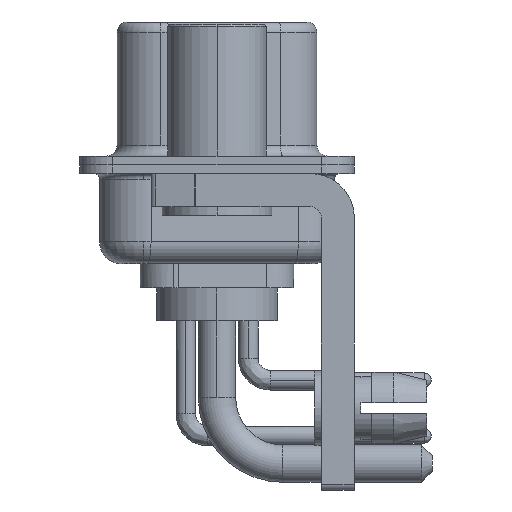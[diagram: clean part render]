
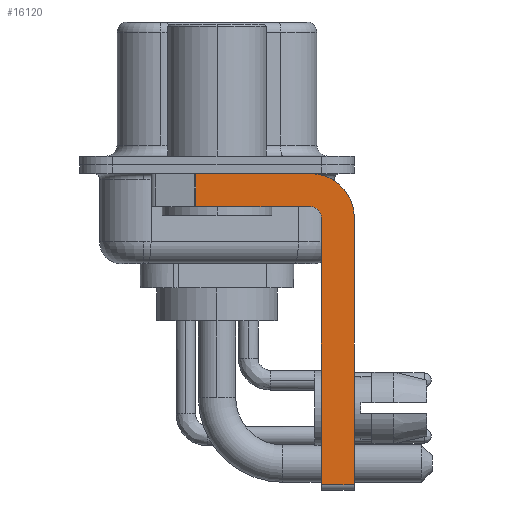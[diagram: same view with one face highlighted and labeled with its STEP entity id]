
A CAD part, left-side view. The second image highlights one B-rep face of the part: STEP entity #16120.
In plain terms, the highlighted planar face has unit normal (-1, 0, 0).
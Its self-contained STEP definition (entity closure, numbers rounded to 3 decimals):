
#442 = PLANE ( 'NONE',  #22238 ) ;
#524 = VECTOR ( 'NONE', #937, 1000. ) ;
#581 = DIRECTION ( 'NONE',  ( 0., 0., -1. ) ) ;
#937 = DIRECTION ( 'NONE',  ( 0., -1., 0. ) ) ;
#1327 = FACE_OUTER_BOUND ( 'NONE', #17227, .T. ) ;
#2246 = EDGE_CURVE ( 'NONE', #13274, #13273, #14665, .T. ) ;
#2663 = CARTESIAN_POINT ( 'NONE',  ( -2.9, -4.75, -2.4 ) ) ;
#3326 = LINE ( 'NONE', #11340, #25984 ) ;
#3501 = EDGE_CURVE ( 'NONE', #24560, #13274, #6571, .T. ) ;
#3505 = CARTESIAN_POINT ( 'NONE',  ( -2.9, -4.75, -14.8 ) ) ;
#3514 = EDGE_CURVE ( 'NONE', #13273, #20298, #10653, .T. ) ;
#4034 = EDGE_CURVE ( 'NONE', #24560, #18613, #13645, .T. ) ;
#4553 = ORIENTED_EDGE ( 'NONE', *, *, #2246, .F. ) ;
#5002 = CARTESIAN_POINT ( 'NONE',  ( -2.9, -6.25, -2.4 ) ) ;
#5004 = DIRECTION ( 'NONE',  ( 1., 0., 0. ) ) ;
#5106 = DIRECTION ( 'NONE',  ( 0., 0., -1. ) ) ;
#5158 = CARTESIAN_POINT ( 'NONE',  ( -2.9, -4.25, -2.4 ) ) ;
#5387 = CARTESIAN_POINT ( 'NONE',  ( -2.9, -4.25, -2.4 ) ) ;
#6396 = VECTOR ( 'NONE', #21031, 1000. ) ;
#6571 = LINE ( 'NONE', #6977, #524 ) ;
#6977 = CARTESIAN_POINT ( 'NONE',  ( -2.9, 3., -0.4 ) ) ;
#7710 = CARTESIAN_POINT ( 'NONE',  ( -2.9, -4.25, -1.9 ) ) ;
#7780 = CARTESIAN_POINT ( 'NONE',  ( -2.9, -4.25, -0.4 ) ) ;
#8499 = EDGE_CURVE ( 'NONE', #9782, #21726, #16261, .T. ) ;
#9782 = VERTEX_POINT ( 'NONE', #2663 ) ;
#10251 = VECTOR ( 'NONE', #13241, 1000. ) ;
#10653 = LINE ( 'NONE', #5002, #6396 ) ;
#10694 = CARTESIAN_POINT ( 'NONE',  ( -2.9, -4.25, -2.4 ) ) ;
#10825 = CARTESIAN_POINT ( 'NONE',  ( -2.9, 0.978, -1.9 ) ) ;
#11340 = CARTESIAN_POINT ( 'NONE',  ( -2.9, -4.25, -1.9 ) ) ;
#12116 = CARTESIAN_POINT ( 'NONE',  ( -2.9, -4.25, -14.55 ) ) ;
#12585 = AXIS2_PLACEMENT_3D ( 'NONE', #5387, #5004, #17216 ) ;
#13179 = DIRECTION ( 'NONE',  ( 0., 0., 1. ) ) ;
#13241 = DIRECTION ( 'NONE',  ( 0., 0., 1. ) ) ;
#13273 = VERTEX_POINT ( 'NONE', #25667 ) ;
#13274 = VERTEX_POINT ( 'NONE', #7780 ) ;
#13645 = LINE ( 'NONE', #19415, #15637 ) ;
#14521 = CARTESIAN_POINT ( 'NONE',  ( -2.9, -4.75, -14.55 ) ) ;
#14626 = EDGE_CURVE ( 'NONE', #21726, #18613, #3326, .T. ) ;
#14665 = CIRCLE ( 'NONE', #12585, 2. ) ;
#14798 = ORIENTED_EDGE ( 'NONE', *, *, #21656, .F. ) ;
#15449 = CARTESIAN_POINT ( 'NONE',  ( -2.9, -6.25, -14.55 ) ) ;
#15452 = LINE ( 'NONE', #3505, #10251 ) ;
#15637 = VECTOR ( 'NONE', #5106, 1000. ) ;
#15831 = AXIS2_PLACEMENT_3D ( 'NONE', #5158, #17366, #13179 ) ;
#16109 = CARTESIAN_POINT ( 'NONE',  ( -2.9, 0.978, -0.4 ) ) ;
#16120 = ADVANCED_FACE ( 'NONE', ( #1327 ), #442, .F. ) ;
#16261 = CIRCLE ( 'NONE', #15831, 0.5 ) ;
#17053 = ORIENTED_EDGE ( 'NONE', *, *, #25625, .T. ) ;
#17216 = DIRECTION ( 'NONE',  ( 0., 0., -1. ) ) ;
#17227 = EDGE_LOOP ( 'NONE', ( #22684, #20893, #23964, #23751, #14798, #17053, #18239, #4553 ) ) ;
#17366 = DIRECTION ( 'NONE',  ( -1., 0., 0. ) ) ;
#17385 = DIRECTION ( 'NONE',  ( 0., 1., 0. ) ) ;
#18239 = ORIENTED_EDGE ( 'NONE', *, *, #3514, .F. ) ;
#18613 = VERTEX_POINT ( 'NONE', #10825 ) ;
#18666 = LINE ( 'NONE', #12116, #22332 ) ;
#19415 = CARTESIAN_POINT ( 'NONE',  ( -2.9, 0.978, -1.9 ) ) ;
#20112 = DIRECTION ( 'NONE',  ( 0., -1., 0. ) ) ;
#20298 = VERTEX_POINT ( 'NONE', #15449 ) ;
#20893 = ORIENTED_EDGE ( 'NONE', *, *, #4034, .T. ) ;
#21031 = DIRECTION ( 'NONE',  ( 0., 0., -1. ) ) ;
#21656 = EDGE_CURVE ( 'NONE', #24717, #9782, #15452, .T. ) ;
#21726 = VERTEX_POINT ( 'NONE', #7710 ) ;
#22238 = AXIS2_PLACEMENT_3D ( 'NONE', #10694, #23399, #581 ) ;
#22332 = VECTOR ( 'NONE', #20112, 1000. ) ;
#22684 = ORIENTED_EDGE ( 'NONE', *, *, #3501, .F. ) ;
#23399 = DIRECTION ( 'NONE',  ( 1., 0., 0. ) ) ;
#23751 = ORIENTED_EDGE ( 'NONE', *, *, #8499, .F. ) ;
#23964 = ORIENTED_EDGE ( 'NONE', *, *, #14626, .F. ) ;
#24560 = VERTEX_POINT ( 'NONE', #16109 ) ;
#24717 = VERTEX_POINT ( 'NONE', #14521 ) ;
#25625 = EDGE_CURVE ( 'NONE', #24717, #20298, #18666, .T. ) ;
#25667 = CARTESIAN_POINT ( 'NONE',  ( -2.9, -6.25, -2.4 ) ) ;
#25984 = VECTOR ( 'NONE', #17385, 1000. ) ;
